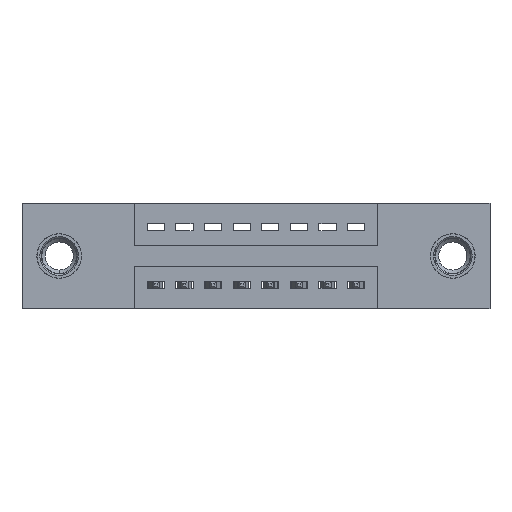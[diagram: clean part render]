
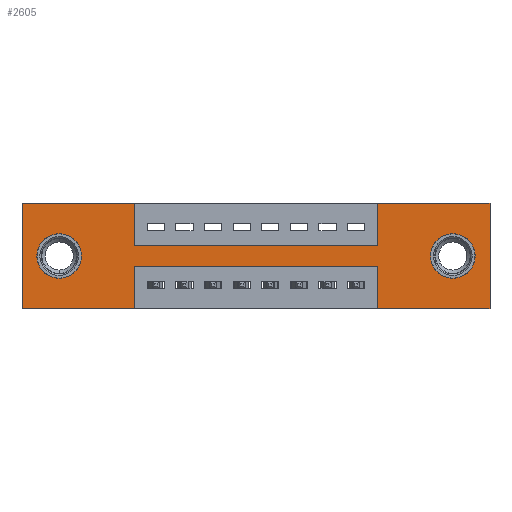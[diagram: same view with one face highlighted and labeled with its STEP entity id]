
A CAD part, front view. The second image highlights one B-rep face of the part: STEP entity #2605.
In plain terms, the highlighted planar face has unit normal (0, -1, 0).
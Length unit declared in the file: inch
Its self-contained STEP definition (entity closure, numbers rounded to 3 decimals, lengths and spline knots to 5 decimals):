
#2 = PLANE ( 'NONE',  #2803 ) ;
#174 = CARTESIAN_POINT ( 'NONE',  ( 1.2425, 0., -0.37 ) ) ;
#206 = ORIENTED_EDGE ( 'NONE', *, *, #627, .T. ) ;
#244 = LINE ( 'NONE', #9438, #6495 ) ;
#291 = ORIENTED_EDGE ( 'NONE', *, *, #11117, .F. ) ;
#293 = CARTESIAN_POINT ( 'NONE',  ( 1.2425, 0., 0. ) ) ;
#338 = VERTEX_POINT ( 'NONE', #6329 ) ;
#403 = DIRECTION ( 'NONE',  ( 1., 0., 0. ) ) ;
#452 = VERTEX_POINT ( 'NONE', #174 ) ;
#476 = LINE ( 'NONE', #8781, #8618 ) ;
#627 = EDGE_CURVE ( 'NONE', #3349, #3415, #6149, .T. ) ;
#692 = LINE ( 'NONE', #8163, #11250 ) ;
#778 = LINE ( 'NONE', #4364, #8336 ) ;
#788 = CARTESIAN_POINT ( 'NONE',  ( 0., 0., -0.37 ) ) ;
#800 = VERTEX_POINT ( 'NONE', #7397 ) ;
#955 = DIRECTION ( 'NONE',  ( -1., 0., 0. ) ) ;
#974 = FACE_OUTER_BOUND ( 'NONE', #3381, .T. ) ;
#1110 = FACE_BOUND ( 'NONE', #2169, .T. ) ;
#1120 = ORIENTED_EDGE ( 'NONE', *, *, #4493, .F. ) ;
#1254 = CARTESIAN_POINT ( 'NONE',  ( 0.13, 0., -0.185 ) ) ;
#1486 = DIRECTION ( 'NONE',  ( -1., 0., 0. ) ) ;
#1524 = EDGE_CURVE ( 'NONE', #452, #10184, #6965, .T. ) ;
#1881 = ORIENTED_EDGE ( 'NONE', *, *, #3273, .F. ) ;
#1893 = CIRCLE ( 'NONE', #4061, 0.078 ) ;
#1954 = CARTESIAN_POINT ( 'NONE',  ( 1.505, 0., -0.263 ) ) ;
#2068 = CARTESIAN_POINT ( 'NONE',  ( 0.3925, 0., 0. ) ) ;
#2077 = VERTEX_POINT ( 'NONE', #3106 ) ;
#2094 = VERTEX_POINT ( 'NONE', #7681 ) ;
#2121 = EDGE_CURVE ( 'NONE', #3424, #9313, #10984, .T. ) ;
#2169 = EDGE_LOOP ( 'NONE', ( #10995, #3345 ) ) ;
#2605 = ADVANCED_FACE ( 'NONE', ( #3064, #1110, #974 ), #2, .T. ) ;
#2611 = VECTOR ( 'NONE', #9014, 39.37008 ) ;
#2650 = CIRCLE ( 'NONE', #3652, 0.078 ) ;
#2667 = EDGE_CURVE ( 'NONE', #9313, #3424, #2650, .T. ) ;
#2696 = DIRECTION ( 'NONE',  ( 1., 0., 0. ) ) ;
#2752 = DIRECTION ( 'NONE',  ( 0., 0., -1. ) ) ;
#2758 = EDGE_CURVE ( 'NONE', #7647, #10065, #3954, .T. ) ;
#2784 = VERTEX_POINT ( 'NONE', #3238 ) ;
#2803 = AXIS2_PLACEMENT_3D ( 'NONE', #10997, #6352, #11037 ) ;
#2869 = CARTESIAN_POINT ( 'NONE',  ( 0.13, 0., -0.107 ) ) ;
#2939 = ORIENTED_EDGE ( 'NONE', *, *, #8376, .F. ) ;
#2987 = DIRECTION ( 'NONE',  ( 0., 1., 0. ) ) ;
#2998 = ORIENTED_EDGE ( 'NONE', *, *, #8661, .F. ) ;
#3003 = CARTESIAN_POINT ( 'NONE',  ( 1.505, 0., -0.185 ) ) ;
#3064 = FACE_BOUND ( 'NONE', #10539, .T. ) ;
#3081 = DIRECTION ( 'NONE',  ( 0., 0., -1. ) ) ;
#3106 = CARTESIAN_POINT ( 'NONE',  ( 0.3925, 0., -0.37 ) ) ;
#3134 = EDGE_CURVE ( 'NONE', #4182, #800, #244, .T. ) ;
#3238 = CARTESIAN_POINT ( 'NONE',  ( 0., 0., 0. ) ) ;
#3273 = EDGE_CURVE ( 'NONE', #2077, #8737, #692, .T. ) ;
#3345 = ORIENTED_EDGE ( 'NONE', *, *, #2667, .T. ) ;
#3348 = LINE ( 'NONE', #9939, #6065 ) ;
#3349 = VERTEX_POINT ( 'NONE', #3916 ) ;
#3381 = EDGE_LOOP ( 'NONE', ( #10048, #2939, #7605, #2998, #6250, #6119, #1120, #291, #6091, #4101, #3943, #1881 ) ) ;
#3415 = VERTEX_POINT ( 'NONE', #1954 ) ;
#3424 = VERTEX_POINT ( 'NONE', #2869 ) ;
#3652 = AXIS2_PLACEMENT_3D ( 'NONE', #1254, #2987, #5692 ) ;
#3689 = CARTESIAN_POINT ( 'NONE',  ( 0., 0., 0. ) ) ;
#3799 = CARTESIAN_POINT ( 'NONE',  ( 0.3925, 0., -0.37 ) ) ;
#3916 = CARTESIAN_POINT ( 'NONE',  ( 1.505, 0., -0.107 ) ) ;
#3943 = ORIENTED_EDGE ( 'NONE', *, *, #8630, .F. ) ;
#3954 = LINE ( 'NONE', #2068, #7236 ) ;
#4061 = AXIS2_PLACEMENT_3D ( 'NONE', #7243, #4633, #2752 ) ;
#4101 = ORIENTED_EDGE ( 'NONE', *, *, #6630, .F. ) ;
#4182 = VERTEX_POINT ( 'NONE', #293 ) ;
#4364 = CARTESIAN_POINT ( 'NONE',  ( 0.3925, 0., -0.22 ) ) ;
#4426 = LINE ( 'NONE', #7185, #10829 ) ;
#4493 = EDGE_CURVE ( 'NONE', #338, #4182, #3348, .T. ) ;
#4633 = DIRECTION ( 'NONE',  ( 0., 1., 0. ) ) ;
#4714 = VECTOR ( 'NONE', #9279, 39.37008 ) ;
#4821 = EDGE_CURVE ( 'NONE', #800, #9634, #6891, .T. ) ;
#4824 = VECTOR ( 'NONE', #6400, 39.37008 ) ;
#4971 = DIRECTION ( 'NONE',  ( 0., 1., 0. ) ) ;
#5304 = EDGE_CURVE ( 'NONE', #3415, #3349, #1893, .T. ) ;
#5470 = CARTESIAN_POINT ( 'NONE',  ( 1.635, 0., 0. ) ) ;
#5637 = DIRECTION ( 'NONE',  ( 0., 0., 1. ) ) ;
#5678 = CARTESIAN_POINT ( 'NONE',  ( 0.13, 0., -0.263 ) ) ;
#5692 = DIRECTION ( 'NONE',  ( 0., 0., 1. ) ) ;
#5721 = CARTESIAN_POINT ( 'NONE',  ( 1.635, 0., -0.37 ) ) ;
#6065 = VECTOR ( 'NONE', #7122, 39.37008 ) ;
#6091 = ORIENTED_EDGE ( 'NONE', *, *, #2758, .F. ) ;
#6119 = ORIENTED_EDGE ( 'NONE', *, *, #3134, .F. ) ;
#6149 = CIRCLE ( 'NONE', #7696, 0.078 ) ;
#6250 = ORIENTED_EDGE ( 'NONE', *, *, #4821, .F. ) ;
#6329 = CARTESIAN_POINT ( 'NONE',  ( 1.2425, 0., -0.15 ) ) ;
#6352 = DIRECTION ( 'NONE',  ( 0., -1., 0. ) ) ;
#6400 = DIRECTION ( 'NONE',  ( 1., 0., 0. ) ) ;
#6495 = VECTOR ( 'NONE', #403, 39.37008 ) ;
#6630 = EDGE_CURVE ( 'NONE', #2784, #7647, #7500, .T. ) ;
#6891 = LINE ( 'NONE', #5470, #2611 ) ;
#6957 = DIRECTION ( 'NONE',  ( -1., 0., 0. ) ) ;
#6965 = LINE ( 'NONE', #8228, #9857 ) ;
#7122 = DIRECTION ( 'NONE',  ( 0., 0., 1. ) ) ;
#7185 = CARTESIAN_POINT ( 'NONE',  ( 0.3925, 0., -0.15 ) ) ;
#7236 = VECTOR ( 'NONE', #7631, 39.37008 ) ;
#7243 = CARTESIAN_POINT ( 'NONE',  ( 1.505, 0., -0.185 ) ) ;
#7397 = CARTESIAN_POINT ( 'NONE',  ( 1.635, 0., 0. ) ) ;
#7500 = LINE ( 'NONE', #3689, #4824 ) ;
#7557 = CARTESIAN_POINT ( 'NONE',  ( 0.13, 0., -0.185 ) ) ;
#7605 = ORIENTED_EDGE ( 'NONE', *, *, #1524, .F. ) ;
#7631 = DIRECTION ( 'NONE',  ( 0., 0., -1. ) ) ;
#7647 = VERTEX_POINT ( 'NONE', #7927 ) ;
#7681 = CARTESIAN_POINT ( 'NONE',  ( 0.3925, 0., -0.22 ) ) ;
#7696 = AXIS2_PLACEMENT_3D ( 'NONE', #3003, #4971, #3081 ) ;
#7927 = CARTESIAN_POINT ( 'NONE',  ( 0.3925, 0., 0. ) ) ;
#7953 = AXIS2_PLACEMENT_3D ( 'NONE', #7557, #10318, #11248 ) ;
#8163 = CARTESIAN_POINT ( 'NONE',  ( 0., 0., -0.37 ) ) ;
#8228 = CARTESIAN_POINT ( 'NONE',  ( 1.2425, 0., -0.37 ) ) ;
#8336 = VECTOR ( 'NONE', #1486, 39.37008 ) ;
#8376 = EDGE_CURVE ( 'NONE', #10184, #2094, #778, .T. ) ;
#8618 = VECTOR ( 'NONE', #10894, 39.37008 ) ;
#8630 = EDGE_CURVE ( 'NONE', #8737, #2784, #476, .T. ) ;
#8661 = EDGE_CURVE ( 'NONE', #9634, #452, #10610, .T. ) ;
#8737 = VERTEX_POINT ( 'NONE', #11158 ) ;
#8781 = CARTESIAN_POINT ( 'NONE',  ( 0., 0., 0. ) ) ;
#8839 = LINE ( 'NONE', #3799, #4714 ) ;
#9014 = DIRECTION ( 'NONE',  ( 0., 0., -1. ) ) ;
#9279 = DIRECTION ( 'NONE',  ( 0., 0., -1. ) ) ;
#9313 = VERTEX_POINT ( 'NONE', #5678 ) ;
#9438 = CARTESIAN_POINT ( 'NONE',  ( 0., 0., 0. ) ) ;
#9634 = VERTEX_POINT ( 'NONE', #5721 ) ;
#9857 = VECTOR ( 'NONE', #5637, 39.37008 ) ;
#9939 = CARTESIAN_POINT ( 'NONE',  ( 1.2425, 0., 0. ) ) ;
#9963 = ORIENTED_EDGE ( 'NONE', *, *, #5304, .T. ) ;
#10048 = ORIENTED_EDGE ( 'NONE', *, *, #10853, .F. ) ;
#10065 = VERTEX_POINT ( 'NONE', #11663 ) ;
#10184 = VERTEX_POINT ( 'NONE', #10581 ) ;
#10318 = DIRECTION ( 'NONE',  ( 0., 1., 0. ) ) ;
#10539 = EDGE_LOOP ( 'NONE', ( #206, #9963 ) ) ;
#10581 = CARTESIAN_POINT ( 'NONE',  ( 1.2425, 0., -0.22 ) ) ;
#10610 = LINE ( 'NONE', #788, #10753 ) ;
#10753 = VECTOR ( 'NONE', #6957, 39.37008 ) ;
#10829 = VECTOR ( 'NONE', #2696, 39.37008 ) ;
#10853 = EDGE_CURVE ( 'NONE', #2094, #2077, #8839, .T. ) ;
#10894 = DIRECTION ( 'NONE',  ( 0., 0., 1. ) ) ;
#10984 = CIRCLE ( 'NONE', #7953, 0.078 ) ;
#10995 = ORIENTED_EDGE ( 'NONE', *, *, #2121, .T. ) ;
#10997 = CARTESIAN_POINT ( 'NONE',  ( 0., 0., -0.37 ) ) ;
#11037 = DIRECTION ( 'NONE',  ( 0., 0., -1. ) ) ;
#11117 = EDGE_CURVE ( 'NONE', #10065, #338, #4426, .T. ) ;
#11158 = CARTESIAN_POINT ( 'NONE',  ( 0., 0., -0.37 ) ) ;
#11248 = DIRECTION ( 'NONE',  ( 0., 0., 1. ) ) ;
#11250 = VECTOR ( 'NONE', #955, 39.37008 ) ;
#11663 = CARTESIAN_POINT ( 'NONE',  ( 0.3925, 0., -0.15 ) ) ;
